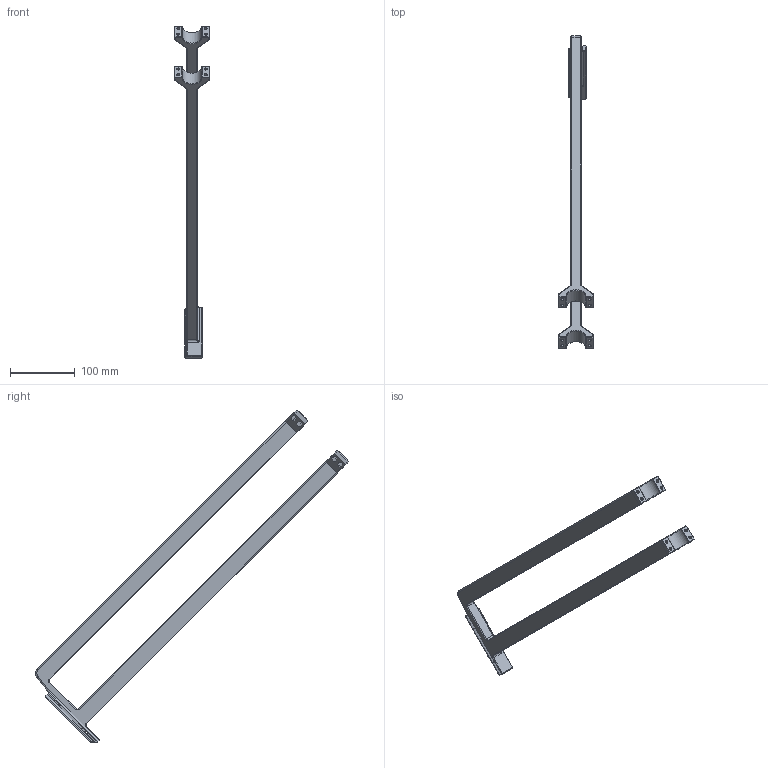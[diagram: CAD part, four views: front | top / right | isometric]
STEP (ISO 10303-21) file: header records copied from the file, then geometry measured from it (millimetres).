
FILE_DESCRIPTION(/* description */ (''),/* implementation_level */ '2;1');
FILE_NAME(/* name */ 'LPL Body - 23in.step',/* time_stamp */ '2022-10-12T08:43:52-05:00',/* author */ (''),/* organization */ (''),/* preprocessor_version */ 'ST-DEVELOPER v19',/* originating_system */ 'Autodesk Translation Framework v11.7.0.108',/* authorisation */ '');
FILE_SCHEMA (('AUTOMOTIVE_DESIGN { 1 0 10303 214 3 1 1 }'));
Length unit declared in the file: millimetre
Products named in the file (1): LPL Optic Mount
Bounding box: 54 x 484.86 x 514.74 mm (x, y, z)
Volume: 512892 mm3; surface area: 109733.7 mm2
Topology: 1 solids, 1 shells, 215 faces, 577 edges, 372 vertices
Faces by surface type: plane 164, cylinder 35, cone 9, bspline 5, torus 2
Full cylindrical faces by diameter (mm): 4.5 x8
Entity records: 7117 total; most frequent: CARTESIAN_POINT 1686, ORIENTED_EDGE 1154, DIRECTION 1050, EDGE_CURVE 577, LINE 462, VECTOR 462, VERTEX_POINT 372, AXIS2_PLACEMENT_3D 294
